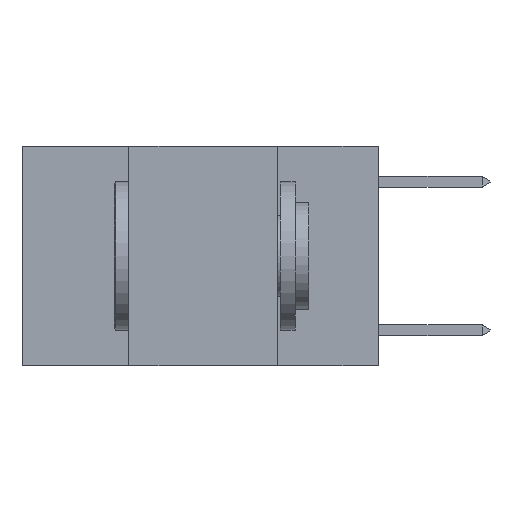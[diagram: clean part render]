
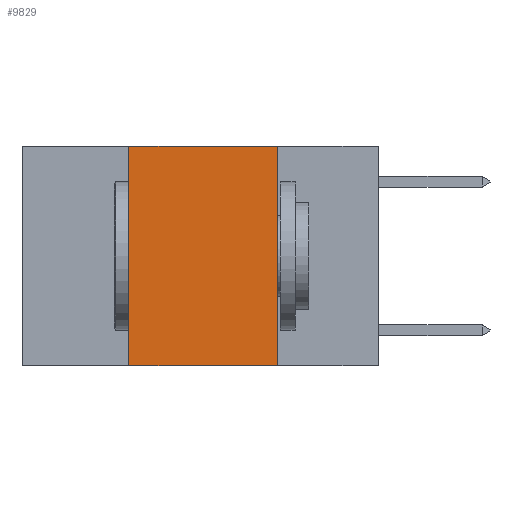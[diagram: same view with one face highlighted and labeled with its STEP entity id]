
A CAD part, left-side view. The second image highlights one B-rep face of the part: STEP entity #9829.
In plain terms, the highlighted planar face has unit normal (-1, 0, 0).
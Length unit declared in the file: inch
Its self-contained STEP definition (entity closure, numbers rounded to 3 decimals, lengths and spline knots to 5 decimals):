
#530 = AXIS2_PLACEMENT_3D ( 'NONE', #7932, #14836, #10659 ) ;
#1418 = VERTEX_POINT ( 'NONE', #10386 ) ;
#1643 = EDGE_LOOP ( 'NONE', ( #16304, #3758, #7846, #13047 ) ) ;
#1824 = CARTESIAN_POINT ( 'NONE',  ( 0., 0.42, -0.37 ) ) ;
#1904 = VERTEX_POINT ( 'NONE', #15972 ) ;
#2336 = LINE ( 'NONE', #5178, #13346 ) ;
#2489 = LINE ( 'NONE', #14320, #10610 ) ;
#2750 = PLANE ( 'NONE',  #530 ) ;
#3758 = ORIENTED_EDGE ( 'NONE', *, *, #7411, .F. ) ;
#4017 = VERTEX_POINT ( 'NONE', #10852 ) ;
#4148 = LINE ( 'NONE', #13197, #7469 ) ;
#5178 = CARTESIAN_POINT ( 'NONE',  ( 0., 0.6, -0.37 ) ) ;
#5223 = EDGE_CURVE ( 'NONE', #16997, #1418, #2336, .T. ) ;
#5462 = DIRECTION ( 'NONE',  ( 0., 0., 1. ) ) ;
#6252 = EDGE_CURVE ( 'NONE', #16997, #1904, #4148, .T. ) ;
#6543 = DIRECTION ( 'NONE',  ( 0., -1., 0. ) ) ;
#7411 = EDGE_CURVE ( 'NONE', #1904, #4017, #2489, .T. ) ;
#7469 = VECTOR ( 'NONE', #5462, 39.37008 ) ;
#7846 = ORIENTED_EDGE ( 'NONE', *, *, #6252, .F. ) ;
#7932 = CARTESIAN_POINT ( 'NONE',  ( 0., 0.6, 0. ) ) ;
#8435 = EDGE_CURVE ( 'NONE', #4017, #1418, #15453, .T. ) ;
#8800 = CARTESIAN_POINT ( 'NONE',  ( 0., 0.17, 0. ) ) ;
#9249 = FACE_OUTER_BOUND ( 'NONE', #1643, .T. ) ;
#9829 = ADVANCED_FACE ( 'NONE', ( #9249 ), #2750, .F. ) ;
#10386 = CARTESIAN_POINT ( 'NONE',  ( 0., 0.17, -0.37 ) ) ;
#10610 = VECTOR ( 'NONE', #16949, 39.37008 ) ;
#10659 = DIRECTION ( 'NONE',  ( 0., 0., -1. ) ) ;
#10852 = CARTESIAN_POINT ( 'NONE',  ( 0., 0.17, 0. ) ) ;
#13047 = ORIENTED_EDGE ( 'NONE', *, *, #5223, .T. ) ;
#13197 = CARTESIAN_POINT ( 'NONE',  ( 0., 0.42, 0. ) ) ;
#13346 = VECTOR ( 'NONE', #6543, 39.37008 ) ;
#14161 = DIRECTION ( 'NONE',  ( 0., 0., -1. ) ) ;
#14320 = CARTESIAN_POINT ( 'NONE',  ( 0., 0.6, 0. ) ) ;
#14836 = DIRECTION ( 'NONE',  ( 1., 0., 0. ) ) ;
#15453 = LINE ( 'NONE', #8800, #15969 ) ;
#15969 = VECTOR ( 'NONE', #14161, 39.37008 ) ;
#15972 = CARTESIAN_POINT ( 'NONE',  ( 0., 0.42, 0. ) ) ;
#16304 = ORIENTED_EDGE ( 'NONE', *, *, #8435, .F. ) ;
#16949 = DIRECTION ( 'NONE',  ( 0., -1., 0. ) ) ;
#16997 = VERTEX_POINT ( 'NONE', #1824 ) ;
